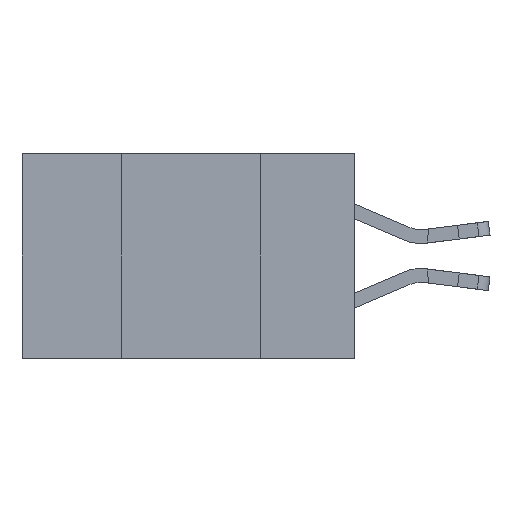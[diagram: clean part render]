
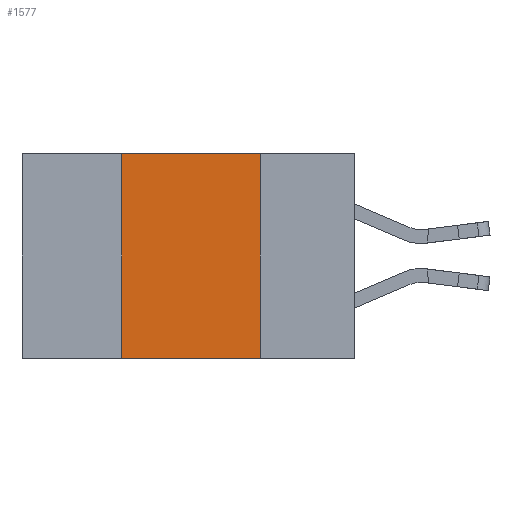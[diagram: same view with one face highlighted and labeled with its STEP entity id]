
A CAD part, left-side view. The second image highlights one B-rep face of the part: STEP entity #1577.
In plain terms, the highlighted planar face has unit normal (-1, 0, 0).
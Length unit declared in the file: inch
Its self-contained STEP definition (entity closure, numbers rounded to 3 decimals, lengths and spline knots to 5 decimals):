
#1130 = VECTOR ( 'NONE', #24884, 39.37008 ) ;
#1577 = ADVANCED_FACE ( 'NONE', ( #17837 ), #22584, .F. ) ;
#1721 = LINE ( 'NONE', #10350, #4880 ) ;
#1751 = LINE ( 'NONE', #7566, #1130 ) ;
#2611 = CARTESIAN_POINT ( 'NONE',  ( 0., 0.6, 0. ) ) ;
#2647 = DIRECTION ( 'NONE',  ( 1., 0., 0. ) ) ;
#3879 = VERTEX_POINT ( 'NONE', #22232 ) ;
#4737 = VERTEX_POINT ( 'NONE', #5547 ) ;
#4748 = EDGE_CURVE ( 'NONE', #24049, #4737, #1721, .T. ) ;
#4788 = VECTOR ( 'NONE', #14832, 39.37008 ) ;
#4880 = VECTOR ( 'NONE', #21721, 39.37008 ) ;
#5547 = CARTESIAN_POINT ( 'NONE',  ( 0., 0.17, 0. ) ) ;
#6410 = EDGE_CURVE ( 'NONE', #4737, #17549, #10660, .T. ) ;
#6688 = ORIENTED_EDGE ( 'NONE', *, *, #10341, .T. ) ;
#7195 = LINE ( 'NONE', #11185, #16965 ) ;
#7566 = CARTESIAN_POINT ( 'NONE',  ( 0., 0.6, -0.37 ) ) ;
#10341 = EDGE_CURVE ( 'NONE', #3879, #17549, #1751, .T. ) ;
#10350 = CARTESIAN_POINT ( 'NONE',  ( 0., 0.6, 0. ) ) ;
#10660 = LINE ( 'NONE', #20639, #4788 ) ;
#11185 = CARTESIAN_POINT ( 'NONE',  ( 0., 0.42, 0. ) ) ;
#11302 = ORIENTED_EDGE ( 'NONE', *, *, #4748, .F. ) ;
#11334 = CARTESIAN_POINT ( 'NONE',  ( 0., 0.42, 0. ) ) ;
#11637 = EDGE_CURVE ( 'NONE', #3879, #24049, #7195, .T. ) ;
#12700 = EDGE_LOOP ( 'NONE', ( #13074, #11302, #17066, #6688 ) ) ;
#13074 = ORIENTED_EDGE ( 'NONE', *, *, #6410, .F. ) ;
#13585 = AXIS2_PLACEMENT_3D ( 'NONE', #2611, #2647, #23573 ) ;
#14832 = DIRECTION ( 'NONE',  ( 0., 0., -1. ) ) ;
#16965 = VECTOR ( 'NONE', #17061, 39.37008 ) ;
#17061 = DIRECTION ( 'NONE',  ( 0., 0., 1. ) ) ;
#17066 = ORIENTED_EDGE ( 'NONE', *, *, #11637, .F. ) ;
#17549 = VERTEX_POINT ( 'NONE', #21258 ) ;
#17837 = FACE_OUTER_BOUND ( 'NONE', #12700, .T. ) ;
#20639 = CARTESIAN_POINT ( 'NONE',  ( 0., 0.17, 0. ) ) ;
#21258 = CARTESIAN_POINT ( 'NONE',  ( 0., 0.17, -0.37 ) ) ;
#21721 = DIRECTION ( 'NONE',  ( 0., -1., 0. ) ) ;
#22232 = CARTESIAN_POINT ( 'NONE',  ( 0., 0.42, -0.37 ) ) ;
#22584 = PLANE ( 'NONE',  #13585 ) ;
#23573 = DIRECTION ( 'NONE',  ( 0., 0., -1. ) ) ;
#24049 = VERTEX_POINT ( 'NONE', #11334 ) ;
#24884 = DIRECTION ( 'NONE',  ( 0., -1., 0. ) ) ;
